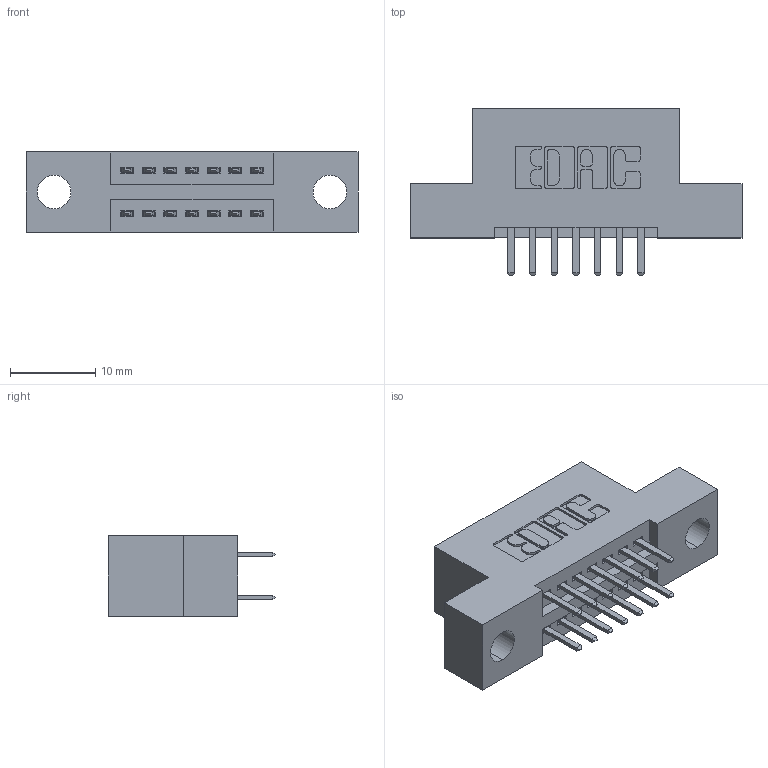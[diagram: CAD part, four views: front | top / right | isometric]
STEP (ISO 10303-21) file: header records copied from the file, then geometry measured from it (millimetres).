
FILE_DESCRIPTION (( 'STEP AP203' ), '1' );
FILE_NAME ('345-014-520-204.STEP', '2018-08-18T07:59:53', ( '' ), ( '' ), 'SwSTEP 2.0', 'SolidWorks 2016', '' );
FILE_SCHEMA (( 'CONFIG_CONTROL_DESIGN' ));
Length unit declared in the file: inch
Products named in the file (3): 345 Part_Flush Mounting Lugs - 0.156 Dia-TH; 345-292-001_345-293-120; 345-014-520-204
Assembly tree (15 placements, depth 2):
  345-014-520-204
    345 Part_Flush Mounting Lugs - 0.156 Dia-TH
    345-292-001_345-293-120  x14
Bounding box: 38.99 x 19.68 x 9.4 mm (x, y, z)
Volume: 3368.5 mm3; surface area: 4103.5 mm2
Topology: 15 solids, 15 shells, 882 faces, 2539 edges, 1654 vertices
Faces by surface type: plane 570, cylinder 312
Entity records: 10321 total; most frequent: CARTESIAN_POINT 1776, ORIENTED_EDGE 1698, DIRECTION 1597, EDGE_CURVE 849, LINE 685, VECTOR 685, VERTEX_POINT 562, AXIS2_PLACEMENT_3D 456
